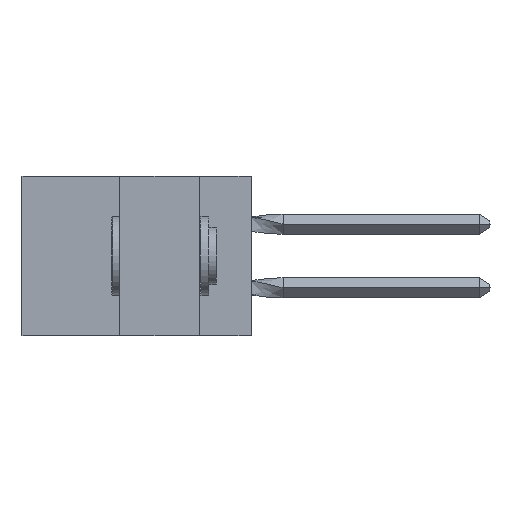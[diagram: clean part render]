
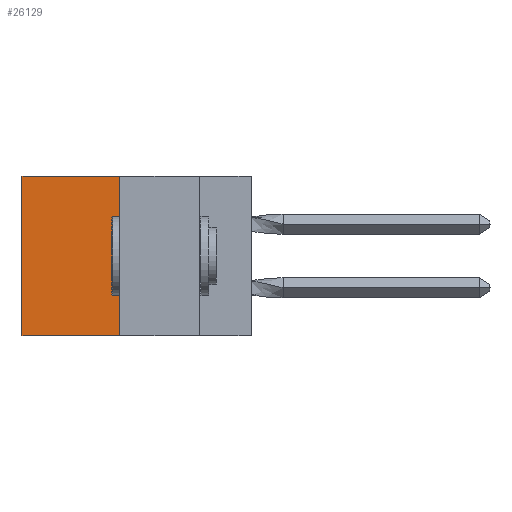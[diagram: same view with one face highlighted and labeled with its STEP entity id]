
A CAD part, left-side view. The second image highlights one B-rep face of the part: STEP entity #26129.
In plain terms, the highlighted planar face has unit normal (-1, 0, 0).
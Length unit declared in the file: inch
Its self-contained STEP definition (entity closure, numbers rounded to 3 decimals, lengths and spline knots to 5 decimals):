
#1345 = CARTESIAN_POINT ( 'NONE',  ( 0.305, 0.413, -0.5 ) ) ;
#3210 = EDGE_CURVE ( 'NONE', #3346, #28022, #9788, .T. ) ;
#3346 = VERTEX_POINT ( 'NONE', #16104 ) ;
#4391 = DIRECTION ( 'NONE',  ( 0., 1., 0. ) ) ;
#4657 = LINE ( 'NONE', #25459, #24590 ) ;
#5166 = DIRECTION ( 'NONE',  ( 1., 0., 0. ) ) ;
#5545 = LINE ( 'NONE', #23285, #19168 ) ;
#6209 = VECTOR ( 'NONE', #4391, 39.37008 ) ;
#6506 = EDGE_CURVE ( 'NONE', #3346, #13158, #4657, .T. ) ;
#7103 = VERTEX_POINT ( 'NONE', #17549 ) ;
#7118 = EDGE_CURVE ( 'NONE', #28022, #7103, #27724, .T. ) ;
#7419 = PLANE ( 'NONE',  #25778 ) ;
#9709 = DIRECTION ( 'NONE',  ( 0., 0., -1. ) ) ;
#9746 = ORIENTED_EDGE ( 'NONE', *, *, #3210, .T. ) ;
#9788 = LINE ( 'NONE', #14197, #6209 ) ;
#10600 = DIRECTION ( 'NONE',  ( 0., 0., -1. ) ) ;
#13158 = VERTEX_POINT ( 'NONE', #1345 ) ;
#13710 = CARTESIAN_POINT ( 'NONE',  ( 0.305, 0.72, 0. ) ) ;
#14197 = CARTESIAN_POINT ( 'NONE',  ( 0.305, 0.413, 0. ) ) ;
#16104 = CARTESIAN_POINT ( 'NONE',  ( 0.305, 0.413, 0. ) ) ;
#16159 = DIRECTION ( 'NONE',  ( 0., 1., 0. ) ) ;
#16333 = CARTESIAN_POINT ( 'NONE',  ( 0.305, 0.413, -0.5 ) ) ;
#16366 = ORIENTED_EDGE ( 'NONE', *, *, #6506, .F. ) ;
#17549 = CARTESIAN_POINT ( 'NONE',  ( 0.305, 0.72, -0.5 ) ) ;
#19168 = VECTOR ( 'NONE', #16159, 39.37008 ) ;
#20167 = EDGE_LOOP ( 'NONE', ( #24211, #27194, #16366, #9746 ) ) ;
#21032 = DIRECTION ( 'NONE',  ( 0., 0., -1. ) ) ;
#22794 = VECTOR ( 'NONE', #10600, 39.37008 ) ;
#23196 = EDGE_CURVE ( 'NONE', #13158, #7103, #5545, .T. ) ;
#23285 = CARTESIAN_POINT ( 'NONE',  ( 0.305, 0.413, -0.5 ) ) ;
#23972 = CARTESIAN_POINT ( 'NONE',  ( 0.305, 0.72, -0.5 ) ) ;
#24211 = ORIENTED_EDGE ( 'NONE', *, *, #7118, .T. ) ;
#24590 = VECTOR ( 'NONE', #21032, 39.37008 ) ;
#25459 = CARTESIAN_POINT ( 'NONE',  ( 0.305, 0.413, -0.5 ) ) ;
#25778 = AXIS2_PLACEMENT_3D ( 'NONE', #16333, #5166, #9709 ) ;
#26129 = ADVANCED_FACE ( 'NONE', ( #27105 ), #7419, .F. ) ;
#27105 = FACE_OUTER_BOUND ( 'NONE', #20167, .T. ) ;
#27194 = ORIENTED_EDGE ( 'NONE', *, *, #23196, .F. ) ;
#27724 = LINE ( 'NONE', #23972, #22794 ) ;
#28022 = VERTEX_POINT ( 'NONE', #13710 ) ;
